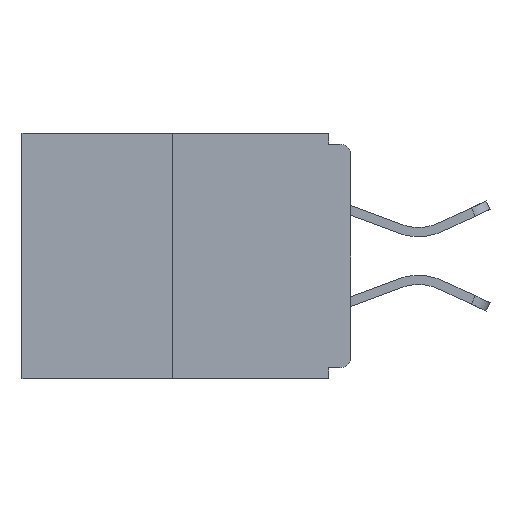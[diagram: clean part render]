
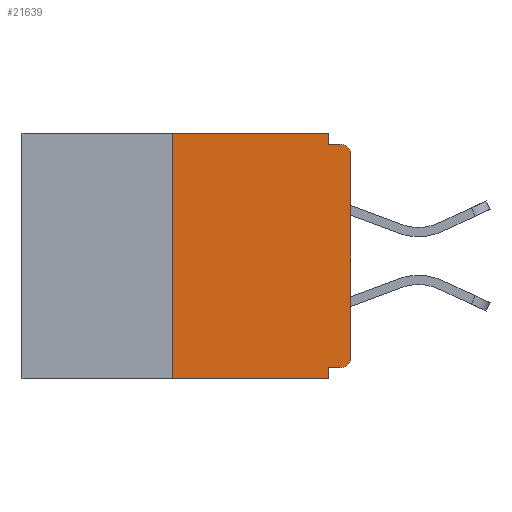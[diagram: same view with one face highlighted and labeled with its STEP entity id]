
A CAD part, left-side view. The second image highlights one B-rep face of the part: STEP entity #21639.
In plain terms, the highlighted planar face has unit normal (-1, 0, 0).
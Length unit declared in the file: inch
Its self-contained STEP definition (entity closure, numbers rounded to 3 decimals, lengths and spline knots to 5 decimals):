
#331 = ORIENTED_EDGE ( 'NONE', *, *, #5544, .T. ) ;
#364 = ORIENTED_EDGE ( 'NONE', *, *, #19873, .F. ) ;
#800 = ORIENTED_EDGE ( 'NONE', *, *, #8507, .T. ) ;
#1376 = LINE ( 'NONE', #21564, #18461 ) ;
#1563 = CARTESIAN_POINT ( 'NONE',  ( 0., 0.031, -0.343 ) ) ;
#1688 = ORIENTED_EDGE ( 'NONE', *, *, #8326, .T. ) ;
#1728 = DIRECTION ( 'NONE',  ( -1., 0., 0. ) ) ;
#1919 = DIRECTION ( 'NONE',  ( 1., 0., 0. ) ) ;
#2353 = VERTEX_POINT ( 'NONE', #22952 ) ;
#2569 = EDGE_CURVE ( 'NONE', #8203, #9409, #16438, .T. ) ;
#2642 = CIRCLE ( 'NONE', #6989, 0.015 ) ;
#2871 = ORIENTED_EDGE ( 'NONE', *, *, #10629, .F. ) ;
#3421 = LINE ( 'NONE', #10227, #22228 ) ;
#3618 = CARTESIAN_POINT ( 'NONE',  ( 0., 0., -0.03 ) ) ;
#3627 = CARTESIAN_POINT ( 'NONE',  ( 0., 0.031, -0.015 ) ) ;
#3707 = FACE_OUTER_BOUND ( 'NONE', #11318, .T. ) ;
#3835 = ORIENTED_EDGE ( 'NONE', *, *, #11602, .F. ) ;
#4167 = VERTEX_POINT ( 'NONE', #4519 ) ;
#4188 = VERTEX_POINT ( 'NONE', #6516 ) ;
#4519 = CARTESIAN_POINT ( 'NONE',  ( 0., 0.015, -0.015 ) ) ;
#4734 = LINE ( 'NONE', #1563, #21262 ) ;
#5544 = EDGE_CURVE ( 'NONE', #23464, #15387, #2642, .T. ) ;
#5598 = CARTESIAN_POINT ( 'NONE',  ( 0., 0., -0.328 ) ) ;
#5698 = CARTESIAN_POINT ( 'NONE',  ( 0., 0.015, -0.328 ) ) ;
#6440 = DIRECTION ( 'NONE',  ( 0., 0., -1. ) ) ;
#6460 = VECTOR ( 'NONE', #17025, 39.37008 ) ;
#6516 = CARTESIAN_POINT ( 'NONE',  ( 0., 0.031, -0.343 ) ) ;
#6678 = CARTESIAN_POINT ( 'NONE',  ( 0., 0.015, -0.03 ) ) ;
#6730 = CIRCLE ( 'NONE', #17519, 0.015 ) ;
#6989 = AXIS2_PLACEMENT_3D ( 'NONE', #21717, #10785, #23547 ) ;
#7263 = CARTESIAN_POINT ( 'NONE',  ( 0., 0.031, 0. ) ) ;
#7277 = ORIENTED_EDGE ( 'NONE', *, *, #18644, .T. ) ;
#7713 = CARTESIAN_POINT ( 'NONE',  ( 0., 0.031, -0.328 ) ) ;
#8039 = VERTEX_POINT ( 'NONE', #11123 ) ;
#8203 = VERTEX_POINT ( 'NONE', #8581 ) ;
#8217 = EDGE_CURVE ( 'NONE', #22447, #4188, #4734, .T. ) ;
#8326 = EDGE_CURVE ( 'NONE', #20755, #4167, #6730, .T. ) ;
#8507 = EDGE_CURVE ( 'NONE', #15387, #20755, #16130, .T. ) ;
#8581 = CARTESIAN_POINT ( 'NONE',  ( 0., 0.031, 0. ) ) ;
#9409 = VERTEX_POINT ( 'NONE', #3627 ) ;
#10103 = DIRECTION ( 'NONE',  ( 0., -1., 0. ) ) ;
#10227 = CARTESIAN_POINT ( 'NONE',  ( 0., 0.25, 0. ) ) ;
#10614 = DIRECTION ( 'NONE',  ( 0., -1., 0. ) ) ;
#10629 = EDGE_CURVE ( 'NONE', #9409, #4167, #11726, .T. ) ;
#10666 = CARTESIAN_POINT ( 'NONE',  ( 0., 0., -0.313 ) ) ;
#10785 = DIRECTION ( 'NONE',  ( -1., 0., 0. ) ) ;
#11123 = CARTESIAN_POINT ( 'NONE',  ( 0., 0.25, 0. ) ) ;
#11318 = EDGE_LOOP ( 'NONE', ( #364, #3835, #7277, #18620, #15337, #331, #800, #1688, #2871, #22389 ) ) ;
#11390 = AXIS2_PLACEMENT_3D ( 'NONE', #22074, #1919, #16476 ) ;
#11602 = EDGE_CURVE ( 'NONE', #2353, #8039, #3421, .T. ) ;
#11726 = LINE ( 'NONE', #22234, #18849 ) ;
#12480 = DIRECTION ( 'NONE',  ( 0., -1., 0. ) ) ;
#14382 = CARTESIAN_POINT ( 'NONE',  ( 0., 0.46, -0.343 ) ) ;
#14574 = DIRECTION ( 'NONE',  ( 0., 0., -1. ) ) ;
#15219 = CARTESIAN_POINT ( 'NONE',  ( 0., 0., 0. ) ) ;
#15337 = ORIENTED_EDGE ( 'NONE', *, *, #19988, .F. ) ;
#15387 = VERTEX_POINT ( 'NONE', #10666 ) ;
#16130 = LINE ( 'NONE', #15219, #6460 ) ;
#16438 = LINE ( 'NONE', #7263, #21572 ) ;
#16476 = DIRECTION ( 'NONE',  ( 0., 0., -1. ) ) ;
#17025 = DIRECTION ( 'NONE',  ( 0., 0., 1. ) ) ;
#17519 = AXIS2_PLACEMENT_3D ( 'NONE', #6678, #1728, #6440 ) ;
#18461 = VECTOR ( 'NONE', #12480, 39.37008 ) ;
#18620 = ORIENTED_EDGE ( 'NONE', *, *, #8217, .F. ) ;
#18644 = EDGE_CURVE ( 'NONE', #2353, #4188, #21384, .T. ) ;
#18849 = VECTOR ( 'NONE', #10103, 39.37008 ) ;
#19873 = EDGE_CURVE ( 'NONE', #8039, #8203, #1376, .T. ) ;
#19888 = LINE ( 'NONE', #5598, #23594 ) ;
#19988 = EDGE_CURVE ( 'NONE', #23464, #22447, #19888, .T. ) ;
#20142 = DIRECTION ( 'NONE',  ( 0., 1., 0. ) ) ;
#20383 = PLANE ( 'NONE',  #11390 ) ;
#20755 = VERTEX_POINT ( 'NONE', #3618 ) ;
#20806 = VECTOR ( 'NONE', #10614, 39.37008 ) ;
#21262 = VECTOR ( 'NONE', #23374, 39.37008 ) ;
#21384 = LINE ( 'NONE', #14382, #20806 ) ;
#21564 = CARTESIAN_POINT ( 'NONE',  ( 0., 0.46, 0. ) ) ;
#21572 = VECTOR ( 'NONE', #14574, 39.37008 ) ;
#21639 = ADVANCED_FACE ( 'NONE', ( #3707 ), #20383, .F. ) ;
#21717 = CARTESIAN_POINT ( 'NONE',  ( 0., 0.015, -0.313 ) ) ;
#22074 = CARTESIAN_POINT ( 'NONE',  ( 0., 0.46, 0. ) ) ;
#22228 = VECTOR ( 'NONE', #22971, 39.37008 ) ;
#22234 = CARTESIAN_POINT ( 'NONE',  ( 0., 0., -0.015 ) ) ;
#22389 = ORIENTED_EDGE ( 'NONE', *, *, #2569, .F. ) ;
#22447 = VERTEX_POINT ( 'NONE', #7713 ) ;
#22952 = CARTESIAN_POINT ( 'NONE',  ( 0., 0.25, -0.343 ) ) ;
#22971 = DIRECTION ( 'NONE',  ( 0., 0., 1. ) ) ;
#23374 = DIRECTION ( 'NONE',  ( 0., 0., -1. ) ) ;
#23464 = VERTEX_POINT ( 'NONE', #5698 ) ;
#23547 = DIRECTION ( 'NONE',  ( 0., 0., -1. ) ) ;
#23594 = VECTOR ( 'NONE', #20142, 39.37008 ) ;
